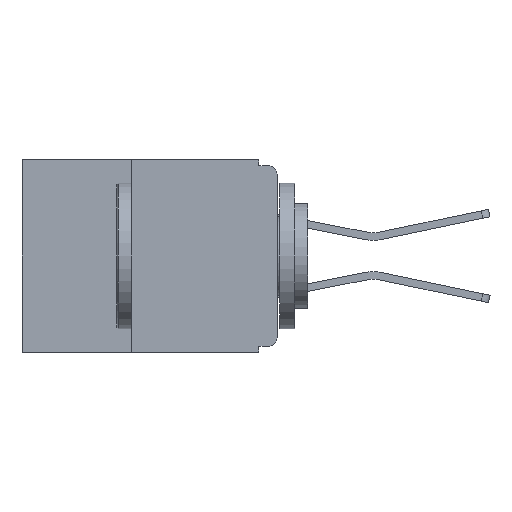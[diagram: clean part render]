
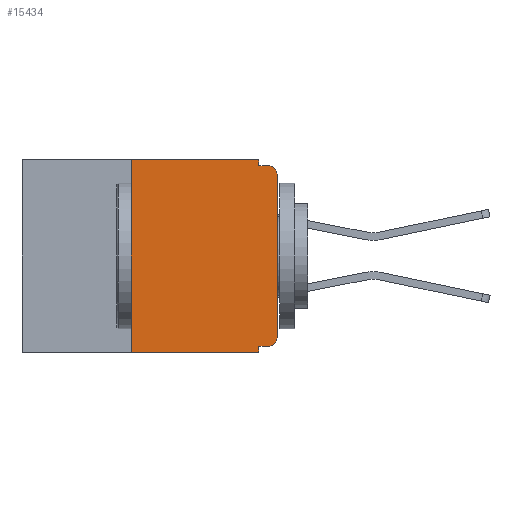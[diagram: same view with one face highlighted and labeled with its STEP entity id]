
A CAD part, left-side view. The second image highlights one B-rep face of the part: STEP entity #15434.
In plain terms, the highlighted planar face has unit normal (-1, 0, 0).
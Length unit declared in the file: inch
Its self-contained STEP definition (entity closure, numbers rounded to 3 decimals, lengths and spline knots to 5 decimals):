
#210 = LINE ( 'NONE', #17235, #11205 ) ;
#362 = DIRECTION ( 'NONE',  ( 0., 0., -1. ) ) ;
#415 = VECTOR ( 'NONE', #8495, 39.37008 ) ;
#786 = VECTOR ( 'NONE', #7203, 39.37008 ) ;
#1316 = EDGE_CURVE ( 'NONE', #15465, #14293, #2700, .T. ) ;
#1533 = ORIENTED_EDGE ( 'NONE', *, *, #17040, .T. ) ;
#1615 = VERTEX_POINT ( 'NONE', #6501 ) ;
#1794 = VECTOR ( 'NONE', #9998, 39.37008 ) ;
#1954 = EDGE_CURVE ( 'NONE', #10926, #13405, #2884, .T. ) ;
#2601 = CARTESIAN_POINT ( 'NONE',  ( 0., 0.25, 0. ) ) ;
#2646 = CARTESIAN_POINT ( 'NONE',  ( 0., 0., -0.32 ) ) ;
#2700 = LINE ( 'NONE', #15451, #9068 ) ;
#2724 = EDGE_CURVE ( 'NONE', #16083, #9196, #12232, .T. ) ;
#2884 = LINE ( 'NONE', #13834, #16802 ) ;
#3069 = VECTOR ( 'NONE', #8366, 39.37008 ) ;
#3168 = ORIENTED_EDGE ( 'NONE', *, *, #4861, .F. ) ;
#3305 = CARTESIAN_POINT ( 'NONE',  ( 0., 0.25, -0.33 ) ) ;
#3366 = ORIENTED_EDGE ( 'NONE', *, *, #2724, .F. ) ;
#3385 = CIRCLE ( 'NONE', #6051, 0.015 ) ;
#3414 = CIRCLE ( 'NONE', #14573, 0.015 ) ;
#4186 = EDGE_CURVE ( 'NONE', #9196, #13405, #210, .T. ) ;
#4266 = DIRECTION ( 'NONE',  ( 1., 0., 0. ) ) ;
#4497 = LINE ( 'NONE', #9942, #786 ) ;
#4582 = ORIENTED_EDGE ( 'NONE', *, *, #1954, .T. ) ;
#4861 = EDGE_CURVE ( 'NONE', #14293, #1615, #11383, .T. ) ;
#5134 = EDGE_CURVE ( 'NONE', #13375, #15465, #10314, .T. ) ;
#5393 = FACE_OUTER_BOUND ( 'NONE', #10264, .T. ) ;
#6051 = AXIS2_PLACEMENT_3D ( 'NONE', #7266, #16700, #8632 ) ;
#6501 = CARTESIAN_POINT ( 'NONE',  ( 0., 0.015, -0.01 ) ) ;
#6512 = CARTESIAN_POINT ( 'NONE',  ( 0., 0.015, -0.025 ) ) ;
#6918 = CARTESIAN_POINT ( 'NONE',  ( 0., 0.437, 0. ) ) ;
#7023 = CARTESIAN_POINT ( 'NONE',  ( 0., 0.031, 0. ) ) ;
#7203 = DIRECTION ( 'NONE',  ( 0., 0., 1. ) ) ;
#7266 = CARTESIAN_POINT ( 'NONE',  ( 0., 0.015, -0.305 ) ) ;
#7374 = LINE ( 'NONE', #9511, #14649 ) ;
#7841 = DIRECTION ( 'NONE',  ( 0., 0., -1. ) ) ;
#8239 = CARTESIAN_POINT ( 'NONE',  ( 0., 0.437, 0. ) ) ;
#8366 = DIRECTION ( 'NONE',  ( 0., -1., 0. ) ) ;
#8495 = DIRECTION ( 'NONE',  ( 0., -1., 0. ) ) ;
#8632 = DIRECTION ( 'NONE',  ( 0., 0., -1. ) ) ;
#8636 = ORIENTED_EDGE ( 'NONE', *, *, #4186, .F. ) ;
#8666 = EDGE_CURVE ( 'NONE', #14121, #13953, #7374, .T. ) ;
#8719 = CARTESIAN_POINT ( 'NONE',  ( 0., 0., -0.01 ) ) ;
#9068 = VECTOR ( 'NONE', #10701, 39.37008 ) ;
#9196 = VERTEX_POINT ( 'NONE', #13246 ) ;
#9356 = CARTESIAN_POINT ( 'NONE',  ( 0., 0., -0.025 ) ) ;
#9511 = CARTESIAN_POINT ( 'NONE',  ( 0., 0., 0. ) ) ;
#9942 = CARTESIAN_POINT ( 'NONE',  ( 0., 0.25, -0.33 ) ) ;
#9998 = DIRECTION ( 'NONE',  ( 0., 1., 0. ) ) ;
#10241 = EDGE_CURVE ( 'NONE', #16083, #14121, #3385, .T. ) ;
#10264 = EDGE_LOOP ( 'NONE', ( #12268, #1533, #3168, #13115, #15638, #12142, #4582, #8636, #3366, #15129 ) ) ;
#10314 = LINE ( 'NONE', #6918, #3069 ) ;
#10701 = DIRECTION ( 'NONE',  ( 0., 0., -1. ) ) ;
#10828 = CARTESIAN_POINT ( 'NONE',  ( 0., 0.031, -0.33 ) ) ;
#10926 = VERTEX_POINT ( 'NONE', #3305 ) ;
#11205 = VECTOR ( 'NONE', #362, 39.37008 ) ;
#11383 = LINE ( 'NONE', #8719, #415 ) ;
#12142 = ORIENTED_EDGE ( 'NONE', *, *, #16739, .F. ) ;
#12232 = LINE ( 'NONE', #2646, #1794 ) ;
#12268 = ORIENTED_EDGE ( 'NONE', *, *, #8666, .T. ) ;
#12421 = PLANE ( 'NONE',  #16270 ) ;
#12452 = CARTESIAN_POINT ( 'NONE',  ( 0., 0.031, -0.01 ) ) ;
#13115 = ORIENTED_EDGE ( 'NONE', *, *, #1316, .F. ) ;
#13246 = CARTESIAN_POINT ( 'NONE',  ( 0., 0.031, -0.32 ) ) ;
#13375 = VERTEX_POINT ( 'NONE', #2601 ) ;
#13405 = VERTEX_POINT ( 'NONE', #10828 ) ;
#13769 = CARTESIAN_POINT ( 'NONE',  ( 0., 0., -0.305 ) ) ;
#13777 = DIRECTION ( 'NONE',  ( 0., 0., -1. ) ) ;
#13834 = CARTESIAN_POINT ( 'NONE',  ( 0., 0.437, -0.33 ) ) ;
#13953 = VERTEX_POINT ( 'NONE', #9356 ) ;
#14121 = VERTEX_POINT ( 'NONE', #13769 ) ;
#14293 = VERTEX_POINT ( 'NONE', #12452 ) ;
#14573 = AXIS2_PLACEMENT_3D ( 'NONE', #6512, #15945, #7841 ) ;
#14649 = VECTOR ( 'NONE', #17471, 39.37008 ) ;
#15129 = ORIENTED_EDGE ( 'NONE', *, *, #10241, .T. ) ;
#15434 = ADVANCED_FACE ( 'NONE', ( #5393 ), #12421, .F. ) ;
#15451 = CARTESIAN_POINT ( 'NONE',  ( 0., 0.031, 0. ) ) ;
#15465 = VERTEX_POINT ( 'NONE', #7023 ) ;
#15638 = ORIENTED_EDGE ( 'NONE', *, *, #5134, .F. ) ;
#15945 = DIRECTION ( 'NONE',  ( -1., 0., 0. ) ) ;
#16083 = VERTEX_POINT ( 'NONE', #16426 ) ;
#16125 = DIRECTION ( 'NONE',  ( 0., -1., 0. ) ) ;
#16270 = AXIS2_PLACEMENT_3D ( 'NONE', #8239, #4266, #13777 ) ;
#16426 = CARTESIAN_POINT ( 'NONE',  ( 0., 0.015, -0.32 ) ) ;
#16700 = DIRECTION ( 'NONE',  ( -1., 0., 0. ) ) ;
#16739 = EDGE_CURVE ( 'NONE', #10926, #13375, #4497, .T. ) ;
#16802 = VECTOR ( 'NONE', #16125, 39.37008 ) ;
#17040 = EDGE_CURVE ( 'NONE', #13953, #1615, #3414, .T. ) ;
#17235 = CARTESIAN_POINT ( 'NONE',  ( 0., 0.031, -0.33 ) ) ;
#17471 = DIRECTION ( 'NONE',  ( 0., 0., 1. ) ) ;
